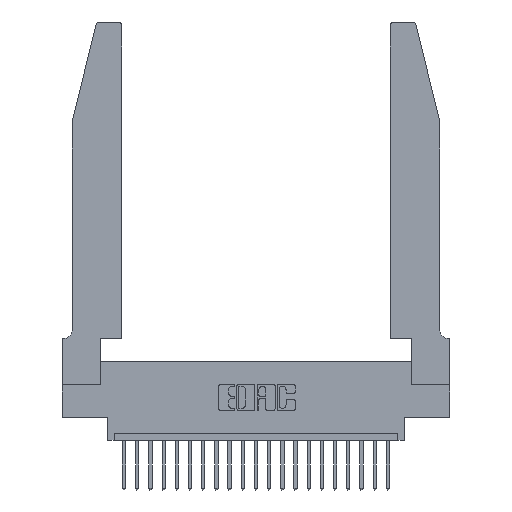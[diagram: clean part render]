
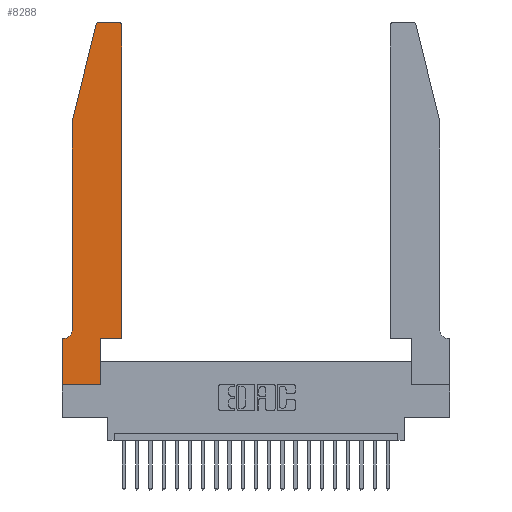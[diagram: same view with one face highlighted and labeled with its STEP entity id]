
A CAD part, top view. The second image highlights one B-rep face of the part: STEP entity #8288.
In plain terms, the highlighted planar face has unit normal (0, 0, 1).
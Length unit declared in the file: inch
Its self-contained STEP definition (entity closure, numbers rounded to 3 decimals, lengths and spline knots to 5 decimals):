
#127 = EDGE_CURVE ( 'NONE', #5945, #20203, #5301, .T. ) ;
#585 = DIRECTION ( 'NONE',  ( 1., 0., 0. ) ) ;
#674 = AXIS2_PLACEMENT_3D ( 'NONE', #8544, #4813, #17659 ) ;
#715 = LINE ( 'NONE', #11133, #16577 ) ;
#1083 = DIRECTION ( 'NONE',  ( 0., -1., 0. ) ) ;
#1523 = DIRECTION ( 'NONE',  ( 1., 0., 0. ) ) ;
#1668 = CARTESIAN_POINT ( 'NONE',  ( 0.0755, 0.35, 0.37 ) ) ;
#1709 = CARTESIAN_POINT ( 'NONE',  ( 0., 0.35, 0.37 ) ) ;
#1894 = LINE ( 'NONE', #1668, #15806 ) ;
#2512 = CARTESIAN_POINT ( 'NONE',  ( 0.4505, 0.35, 0.37 ) ) ;
#2621 = VERTEX_POINT ( 'NONE', #13263 ) ;
#3079 = CARTESIAN_POINT ( 'NONE',  ( 0.0755, 2., 0.37 ) ) ;
#3314 = CARTESIAN_POINT ( 'NONE',  ( 0.2865, 0., 0.37 ) ) ;
#3646 = DIRECTION ( 'NONE',  ( 0., 0., 1. ) ) ;
#3656 = VECTOR ( 'NONE', #1083, 39.37008 ) ;
#3743 = EDGE_LOOP ( 'NONE', ( #7662, #8177, #5318, #7779, #13264, #14257, #19609, #21661, #10133, #18458, #18090, #9370 ) ) ;
#4139 = CARTESIAN_POINT ( 'NONE',  ( 0.2605, 2.75, 0.37 ) ) ;
#4525 = DIRECTION ( 'NONE',  ( 0., 1., 0. ) ) ;
#4719 = EDGE_CURVE ( 'NONE', #11627, #12134, #17612, .T. ) ;
#4813 = DIRECTION ( 'NONE',  ( 0., 0., 1. ) ) ;
#4864 = CARTESIAN_POINT ( 'NONE',  ( 0.0755, 2., 0.37 ) ) ;
#5301 = LINE ( 'NONE', #4864, #12980 ) ;
#5318 = ORIENTED_EDGE ( 'NONE', *, *, #127, .T. ) ;
#5499 = CIRCLE ( 'NONE', #674, 0.03 ) ;
#5670 = CARTESIAN_POINT ( 'NONE',  ( 0., 0., 0.37 ) ) ;
#5772 = VERTEX_POINT ( 'NONE', #3314 ) ;
#5870 = DIRECTION ( 'NONE',  ( 0., 1., 0. ) ) ;
#5945 = VERTEX_POINT ( 'NONE', #17162 ) ;
#6214 = CARTESIAN_POINT ( 'NONE',  ( 0.0755, 2., 0.37 ) ) ;
#6836 = AXIS2_PLACEMENT_3D ( 'NONE', #1709, #3646, #16301 ) ;
#6995 = DIRECTION ( 'NONE',  ( 0., -1., 0. ) ) ;
#7550 = CARTESIAN_POINT ( 'NONE',  ( 0., 0.35, 0.37 ) ) ;
#7662 = ORIENTED_EDGE ( 'NONE', *, *, #20064, .T. ) ;
#7714 = DIRECTION ( 'NONE',  ( -1., 0., 0. ) ) ;
#7779 = ORIENTED_EDGE ( 'NONE', *, *, #18313, .T. ) ;
#7862 = EDGE_CURVE ( 'NONE', #2621, #11827, #715, .T. ) ;
#8049 = LINE ( 'NONE', #13104, #16520 ) ;
#8177 = ORIENTED_EDGE ( 'NONE', *, *, #19139, .T. ) ;
#8288 = ADVANCED_FACE ( 'NONE', ( #11469 ), #19980, .T. ) ;
#8544 = CARTESIAN_POINT ( 'NONE',  ( 0.4205, 2.72, 0.37 ) ) ;
#8934 = LINE ( 'NONE', #4139, #20583 ) ;
#9237 = LINE ( 'NONE', #15250, #15759 ) ;
#9369 = CARTESIAN_POINT ( 'NONE',  ( 0., 0., 0.37 ) ) ;
#9370 = ORIENTED_EDGE ( 'NONE', *, *, #14567, .T. ) ;
#9737 = EDGE_CURVE ( 'NONE', #9935, #22580, #16794, .T. ) ;
#9935 = VERTEX_POINT ( 'NONE', #7550 ) ;
#10133 = ORIENTED_EDGE ( 'NONE', *, *, #21125, .T. ) ;
#10827 = DIRECTION ( 'NONE',  ( 0., 0., -1. ) ) ;
#11133 = CARTESIAN_POINT ( 'NONE',  ( 0.4505, 0.35, 0.37 ) ) ;
#11469 = FACE_OUTER_BOUND ( 'NONE', #3743, .T. ) ;
#11627 = VERTEX_POINT ( 'NONE', #20179 ) ;
#11827 = VERTEX_POINT ( 'NONE', #2512 ) ;
#12134 = VERTEX_POINT ( 'NONE', #23036 ) ;
#12399 = DIRECTION ( 'NONE',  ( 0., 0., 1. ) ) ;
#12980 = VECTOR ( 'NONE', #18836, 39.37008 ) ;
#13104 = CARTESIAN_POINT ( 'NONE',  ( 0.2865, 0.35, 0.37 ) ) ;
#13173 = CARTESIAN_POINT ( 'NONE',  ( 0.4505, 0.35, 0.37 ) ) ;
#13263 = CARTESIAN_POINT ( 'NONE',  ( 0.2865, 0.35, 0.37 ) ) ;
#13264 = ORIENTED_EDGE ( 'NONE', *, *, #4719, .T. ) ;
#13823 = AXIS2_PLACEMENT_3D ( 'NONE', #23286, #12399, #1523 ) ;
#14257 = ORIENTED_EDGE ( 'NONE', *, *, #18743, .T. ) ;
#14391 = VECTOR ( 'NONE', #5870, 39.37008 ) ;
#14567 = EDGE_CURVE ( 'NONE', #19544, #18540, #5499, .T. ) ;
#15250 = CARTESIAN_POINT ( 'NONE',  ( 0., 0., 0.37 ) ) ;
#15260 = LINE ( 'NONE', #13173, #14391 ) ;
#15759 = VECTOR ( 'NONE', #585, 39.37008 ) ;
#15806 = VECTOR ( 'NONE', #19694, 39.37008 ) ;
#16301 = DIRECTION ( 'NONE',  ( 1., 0., 0. ) ) ;
#16520 = VECTOR ( 'NONE', #4525, 39.37008 ) ;
#16577 = VECTOR ( 'NONE', #18533, 39.37008 ) ;
#16721 = CARTESIAN_POINT ( 'NONE',  ( 0.4205, 2.75, 0.37 ) ) ;
#16794 = LINE ( 'NONE', #5670, #21348 ) ;
#17162 = CARTESIAN_POINT ( 'NONE',  ( 0.25487, 2.72718, 0.37 ) ) ;
#17612 = CIRCLE ( 'NONE', #19680, 0.07 ) ;
#17659 = DIRECTION ( 'NONE',  ( 1., 0., 0. ) ) ;
#18090 = ORIENTED_EDGE ( 'NONE', *, *, #23136, .T. ) ;
#18313 = EDGE_CURVE ( 'NONE', #20203, #11627, #21802, .T. ) ;
#18458 = ORIENTED_EDGE ( 'NONE', *, *, #7862, .T. ) ;
#18533 = DIRECTION ( 'NONE',  ( 1., 0., 0. ) ) ;
#18540 = VERTEX_POINT ( 'NONE', #16721 ) ;
#18743 = EDGE_CURVE ( 'NONE', #12134, #9935, #1894, .T. ) ;
#18836 = DIRECTION ( 'NONE',  ( -0.239, -0.971, 0. ) ) ;
#19139 = EDGE_CURVE ( 'NONE', #20587, #5945, #20917, .T. ) ;
#19544 = VERTEX_POINT ( 'NONE', #23161 ) ;
#19609 = ORIENTED_EDGE ( 'NONE', *, *, #9737, .T. ) ;
#19615 = EDGE_CURVE ( 'NONE', #22580, #5772, #9237, .T. ) ;
#19680 = AXIS2_PLACEMENT_3D ( 'NONE', #23457, #10827, #7714 ) ;
#19694 = DIRECTION ( 'NONE',  ( -1., 0., 0. ) ) ;
#19980 = PLANE ( 'NONE',  #6836 ) ;
#20064 = EDGE_CURVE ( 'NONE', #18540, #20587, #8934, .T. ) ;
#20136 = CARTESIAN_POINT ( 'NONE',  ( 0.284, 2.75, 0.37 ) ) ;
#20179 = CARTESIAN_POINT ( 'NONE',  ( 0.0755, 0.42, 0.37 ) ) ;
#20203 = VERTEX_POINT ( 'NONE', #6214 ) ;
#20322 = DIRECTION ( 'NONE',  ( -1., 0., 0. ) ) ;
#20583 = VECTOR ( 'NONE', #20322, 39.37008 ) ;
#20587 = VERTEX_POINT ( 'NONE', #20136 ) ;
#20917 = CIRCLE ( 'NONE', #13823, 0.03 ) ;
#21125 = EDGE_CURVE ( 'NONE', #5772, #2621, #8049, .T. ) ;
#21348 = VECTOR ( 'NONE', #6995, 39.37008 ) ;
#21661 = ORIENTED_EDGE ( 'NONE', *, *, #19615, .T. ) ;
#21802 = LINE ( 'NONE', #3079, #3656 ) ;
#22580 = VERTEX_POINT ( 'NONE', #9369 ) ;
#23036 = CARTESIAN_POINT ( 'NONE',  ( 0.0055, 0.35, 0.37 ) ) ;
#23136 = EDGE_CURVE ( 'NONE', #11827, #19544, #15260, .T. ) ;
#23161 = CARTESIAN_POINT ( 'NONE',  ( 0.4505, 2.72, 0.37 ) ) ;
#23286 = CARTESIAN_POINT ( 'NONE',  ( 0.284, 2.72, 0.37 ) ) ;
#23457 = CARTESIAN_POINT ( 'NONE',  ( 0.0055, 0.42, 0.37 ) ) ;
